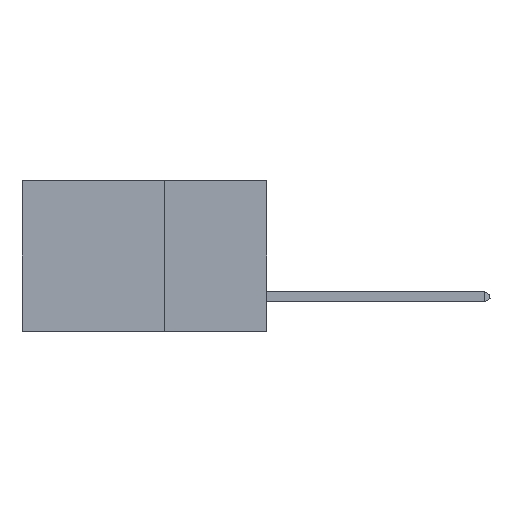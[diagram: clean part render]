
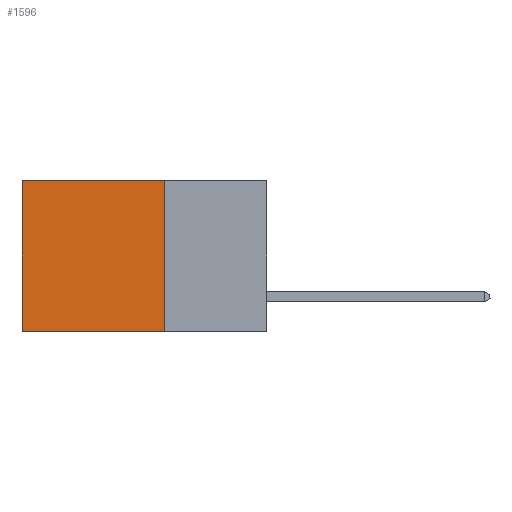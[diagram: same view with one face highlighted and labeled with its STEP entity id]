
A CAD part, left-side view. The second image highlights one B-rep face of the part: STEP entity #1596.
In plain terms, the highlighted planar face has unit normal (-1, 0, 0).
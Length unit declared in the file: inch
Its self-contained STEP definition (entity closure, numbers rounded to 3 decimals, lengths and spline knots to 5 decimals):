
#834 = ORIENTED_EDGE ( 'NONE', *, *, #25692, .F. ) ;
#841 = CARTESIAN_POINT ( 'NONE',  ( 0.2875, 0.25, 0. ) ) ;
#1005 = DIRECTION ( 'NONE',  ( 0., 1., 0. ) ) ;
#1596 = ADVANCED_FACE ( 'NONE', ( #17415 ), #10042, .F. ) ;
#1721 = DIRECTION ( 'NONE',  ( 1., 0., 0. ) ) ;
#5180 = LINE ( 'NONE', #26086, #21688 ) ;
#6666 = LINE ( 'NONE', #7145, #25545 ) ;
#7145 = CARTESIAN_POINT ( 'NONE',  ( 0.2875, 0.6, 0. ) ) ;
#7437 = DIRECTION ( 'NONE',  ( 0., 0., -1. ) ) ;
#7966 = ORIENTED_EDGE ( 'NONE', *, *, #16569, .T. ) ;
#8064 = VECTOR ( 'NONE', #1005, 39.37008 ) ;
#9651 = LINE ( 'NONE', #841, #23818 ) ;
#10042 = PLANE ( 'NONE',  #13806 ) ;
#10394 = CARTESIAN_POINT ( 'NONE',  ( 0.2875, 0.25, 0. ) ) ;
#11091 = EDGE_CURVE ( 'NONE', #17757, #21970, #6666, .T. ) ;
#11591 = EDGE_CURVE ( 'NONE', #27294, #19620, #9651, .T. ) ;
#11719 = CARTESIAN_POINT ( 'NONE',  ( 0.2875, 0.25, 0. ) ) ;
#12971 = DIRECTION ( 'NONE',  ( 0., 1., 0. ) ) ;
#13806 = AXIS2_PLACEMENT_3D ( 'NONE', #20957, #1721, #25101 ) ;
#14137 = ORIENTED_EDGE ( 'NONE', *, *, #11091, .T. ) ;
#15175 = ORIENTED_EDGE ( 'NONE', *, *, #11591, .F. ) ;
#16493 = CARTESIAN_POINT ( 'NONE',  ( 0.2875, 0.6, 0. ) ) ;
#16569 = EDGE_CURVE ( 'NONE', #27294, #17757, #27251, .T. ) ;
#17415 = FACE_OUTER_BOUND ( 'NONE', #22663, .T. ) ;
#17757 = VERTEX_POINT ( 'NONE', #16493 ) ;
#19502 = CARTESIAN_POINT ( 'NONE',  ( 0.2875, 0.6, -0.37 ) ) ;
#19620 = VERTEX_POINT ( 'NONE', #25972 ) ;
#20957 = CARTESIAN_POINT ( 'NONE',  ( 0.2875, 0.25, 0. ) ) ;
#21688 = VECTOR ( 'NONE', #12971, 39.37008 ) ;
#21970 = VERTEX_POINT ( 'NONE', #19502 ) ;
#22663 = EDGE_LOOP ( 'NONE', ( #14137, #834, #15175, #7966 ) ) ;
#23818 = VECTOR ( 'NONE', #7437, 39.37008 ) ;
#24554 = DIRECTION ( 'NONE',  ( 0., 0., -1. ) ) ;
#25101 = DIRECTION ( 'NONE',  ( 0., 0., -1. ) ) ;
#25545 = VECTOR ( 'NONE', #24554, 39.37008 ) ;
#25692 = EDGE_CURVE ( 'NONE', #19620, #21970, #5180, .T. ) ;
#25972 = CARTESIAN_POINT ( 'NONE',  ( 0.2875, 0.25, -0.37 ) ) ;
#26086 = CARTESIAN_POINT ( 'NONE',  ( 0.2875, 0.25, -0.37 ) ) ;
#27251 = LINE ( 'NONE', #11719, #8064 ) ;
#27294 = VERTEX_POINT ( 'NONE', #10394 ) ;
